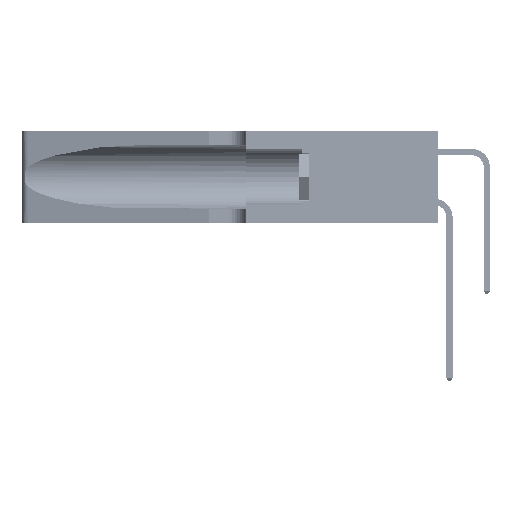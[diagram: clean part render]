
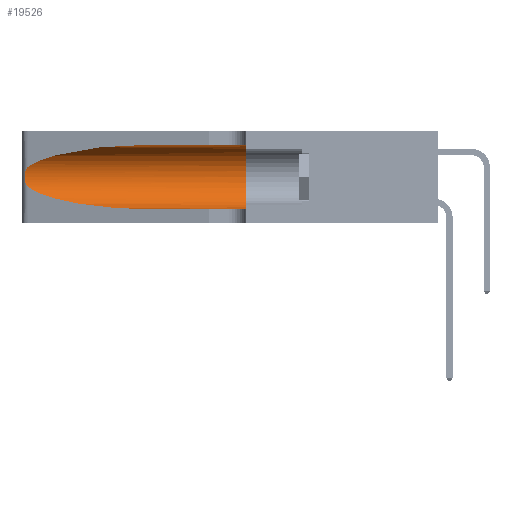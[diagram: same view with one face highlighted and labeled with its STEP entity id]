
A CAD part, left-side view. The second image highlights one B-rep face of the part: STEP entity #19526.
In plain terms, the highlighted cylindrical face has radius 3.308 mm (diameter 6.617 mm), a partial arc.
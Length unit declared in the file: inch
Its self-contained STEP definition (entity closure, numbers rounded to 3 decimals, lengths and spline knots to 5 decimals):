
#2416 = EDGE_CURVE ( 'NONE', #39642, #27867, #42770, .T. ) ;
#2959 = CARTESIAN_POINT ( 'NONE',  ( 0.2373, 1.15595, 0.08982 ) ) ;
#3236 = CARTESIAN_POINT ( 'NONE',  ( 0.25555, 1.22994, 0.2215 ) ) ;
#3404 = CARTESIAN_POINT ( 'NONE',  ( 0.26075, 1.23896, 0.178 ) ) ;
#4704 = VERTEX_POINT ( 'NONE', #21809 ) ;
#5931 = CYLINDRICAL_SURFACE ( 'NONE', #10976, 0.13025 ) ;
#7535 = CARTESIAN_POINT ( 'NONE',  ( 0.25856, 1.23593, 0.16098 ) ) ;
#9279 = ORIENTED_EDGE ( 'NONE', *, *, #2416, .F. ) ;
#10097 = AXIS2_PLACEMENT_3D ( 'NONE', #39865, #15671, #43930 ) ;
#10976 = AXIS2_PLACEMENT_3D ( 'NONE', #12491, #40799, #44662 ) ;
#11651 = CARTESIAN_POINT ( 'NONE',  ( 0.25639, 1.23186, 0.15144 ) ) ;
#12468 = B_SPLINE_CURVE_WITH_KNOTS ( 'NONE', 3,
 ( #35729, #3236, #19637, #47865, #23709, #51926, #27773, #3404, #31870, #7535, #35897, #11651, #39942, #15739 ),
 .UNSPECIFIED., .F., .F.,
 ( 4, 2, 2, 2, 2, 2, 4 ),
 ( 0., 0.00027, 0.00053, 0.00107, 0.0016, 0.00187, 0.00214 ),
 .UNSPECIFIED. ) ;
#12491 = CARTESIAN_POINT ( 'NONE',  ( 0.1305, 1.61858, 0.185 ) ) ;
#13606 = EDGE_CURVE ( 'NONE', #27867, #25632, #39226, .T. ) ;
#15671 = DIRECTION ( 'NONE',  ( 0., 1., 0. ) ) ;
#15739 = CARTESIAN_POINT ( 'NONE',  ( 0.25487, 1.22718, 0.14631 ) ) ;
#15959 = EDGE_CURVE ( 'NONE', #39642, #20517, #16366, .T. ) ;
#16002 = CARTESIAN_POINT ( 'NONE',  ( 0.25487, 1.22718, 0.14631 ) ) ;
#16366 =( BOUNDED_CURVE ( )  B_SPLINE_CURVE ( 3, ( #17527, #29573, #37692, #21599 ),
 .UNSPECIFIED., .F., .F. ) 
 B_SPLINE_CURVE_WITH_KNOTS ( ( 4, 4 ),
 ( 1.5708, 2.84003 ),
 .UNSPECIFIED. ) 
 CURVE ( )  GEOMETRIC_REPRESENTATION_ITEM ( )  RATIONAL_B_SPLINE_CURVE ( ( 1., 0.87, 0.87, 1. ) ) 
 REPRESENTATION_ITEM ( '' )  );
#16986 = EDGE_LOOP ( 'NONE', ( #23969, #51104, #46017, #28983, #38484, #9279 ) ) ;
#17527 = CARTESIAN_POINT ( 'NONE',  ( 0.1305, 0.72297, 0.31525 ) ) ;
#19526 = ADVANCED_FACE ( 'NONE', ( #38301 ), #5931, .F. ) ;
#19637 = CARTESIAN_POINT ( 'NONE',  ( 0.25639, 1.23184, 0.21858 ) ) ;
#19972 = DIRECTION ( 'NONE',  ( 0., -1., 0. ) ) ;
#20517 = VERTEX_POINT ( 'NONE', #38537 ) ;
#21599 = CARTESIAN_POINT ( 'NONE',  ( 0.25487, 1.22718, 0.22369 ) ) ;
#21809 = CARTESIAN_POINT ( 'NONE',  ( 0.1305, 0.72297, 0.05475 ) ) ;
#22747 = CARTESIAN_POINT ( 'NONE',  ( 0.1305, 0.35, 0.31525 ) ) ;
#23450 = CARTESIAN_POINT ( 'NONE',  ( 0.18966, 0.96281, 0.05475 ) ) ;
#23709 = CARTESIAN_POINT ( 'NONE',  ( 0.25854, 1.2359, 0.20912 ) ) ;
#23967 = VERTEX_POINT ( 'NONE', #16002 ) ;
#23969 = ORIENTED_EDGE ( 'NONE', *, *, #15959, .T. ) ;
#24553 = DIRECTION ( 'NONE',  ( 0., -1., 0. ) ) ;
#25084 = EDGE_CURVE ( 'NONE', #4704, #25632, #49280, .T. ) ;
#25632 = VERTEX_POINT ( 'NONE', #39367 ) ;
#27773 = CARTESIAN_POINT ( 'NONE',  ( 0.26075, 1.23896, 0.19203 ) ) ;
#27867 = VERTEX_POINT ( 'NONE', #22747 ) ;
#28666 = EDGE_CURVE ( 'NONE', #20517, #23967, #12468, .T. ) ;
#28983 = ORIENTED_EDGE ( 'NONE', *, *, #25084, .T. ) ;
#29573 = CARTESIAN_POINT ( 'NONE',  ( 0.18966, 0.96281, 0.31525 ) ) ;
#31870 = CARTESIAN_POINT ( 'NONE',  ( 0.26017, 1.23833, 0.17102 ) ) ;
#35729 = CARTESIAN_POINT ( 'NONE',  ( 0.25487, 1.22718, 0.22369 ) ) ;
#35897 = CARTESIAN_POINT ( 'NONE',  ( 0.25789, 1.23486, 0.15765 ) ) ;
#37692 = CARTESIAN_POINT ( 'NONE',  ( 0.2373, 1.15595, 0.28018 ) ) ;
#38301 = FACE_OUTER_BOUND ( 'NONE', #16986, .T. ) ;
#38484 = ORIENTED_EDGE ( 'NONE', *, *, #13606, .F. ) ;
#38537 = CARTESIAN_POINT ( 'NONE',  ( 0.25487, 1.22718, 0.22369 ) ) ;
#39226 = CIRCLE ( 'NONE', #10097, 0.13025 ) ;
#39367 = CARTESIAN_POINT ( 'NONE',  ( 0.1305, 0.35, 0.05475 ) ) ;
#39526 = CARTESIAN_POINT ( 'NONE',  ( 0.25487, 1.22718, 0.14631 ) ) ;
#39642 = VERTEX_POINT ( 'NONE', #39905 ) ;
#39865 = CARTESIAN_POINT ( 'NONE',  ( 0.1305, 0.35, 0.185 ) ) ;
#39905 = CARTESIAN_POINT ( 'NONE',  ( 0.1305, 0.72297, 0.31525 ) ) ;
#39942 = CARTESIAN_POINT ( 'NONE',  ( 0.25555, 1.22993, 0.14849 ) ) ;
#40105 = CARTESIAN_POINT ( 'NONE',  ( 0.1305, 1.61858, 0.05475 ) ) ;
#40799 = DIRECTION ( 'NONE',  ( 0., -1., 0. ) ) ;
#42284 =( BOUNDED_CURVE ( )  B_SPLINE_CURVE ( 3, ( #39526, #2959, #23450, #51661 ),
 .UNSPECIFIED., .F., .T. ) 
 B_SPLINE_CURVE_WITH_KNOTS ( ( 4, 4 ),
 ( 3.44316, 4.71239 ),
 .UNSPECIFIED. ) 
 CURVE ( )  GEOMETRIC_REPRESENTATION_ITEM ( )  RATIONAL_B_SPLINE_CURVE ( ( 1., 0.87, 0.87, 1. ) ) 
 REPRESENTATION_ITEM ( '' )  );
#42770 = LINE ( 'NONE', #48726, #45268 ) ;
#43930 = DIRECTION ( 'NONE',  ( 0., 0., 1. ) ) ;
#44662 = DIRECTION ( 'NONE',  ( 0., 0., -1. ) ) ;
#45268 = VECTOR ( 'NONE', #24553, 39.37008 ) ;
#46017 = ORIENTED_EDGE ( 'NONE', *, *, #47679, .T. ) ;
#47679 = EDGE_CURVE ( 'NONE', #23967, #4704, #42284, .T. ) ;
#47865 = CARTESIAN_POINT ( 'NONE',  ( 0.25787, 1.23484, 0.2124 ) ) ;
#48020 = VECTOR ( 'NONE', #19972, 39.37008 ) ;
#48726 = CARTESIAN_POINT ( 'NONE',  ( 0.1305, 1.61858, 0.31525 ) ) ;
#49280 = LINE ( 'NONE', #40105, #48020 ) ;
#51104 = ORIENTED_EDGE ( 'NONE', *, *, #28666, .T. ) ;
#51661 = CARTESIAN_POINT ( 'NONE',  ( 0.1305, 0.72297, 0.05475 ) ) ;
#51926 = CARTESIAN_POINT ( 'NONE',  ( 0.26018, 1.23835, 0.19895 ) ) ;
